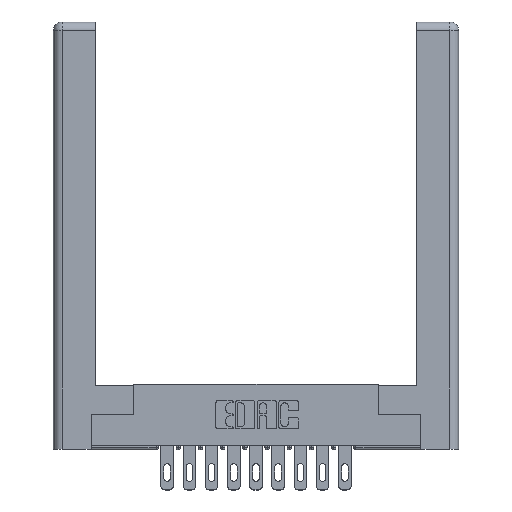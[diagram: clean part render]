
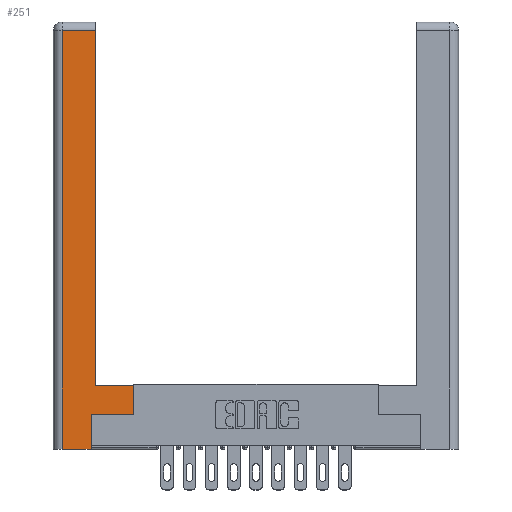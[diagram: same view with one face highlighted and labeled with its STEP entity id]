
A CAD part, top view. The second image highlights one B-rep face of the part: STEP entity #251.
In plain terms, the highlighted planar face has unit normal (0, 0, 1).
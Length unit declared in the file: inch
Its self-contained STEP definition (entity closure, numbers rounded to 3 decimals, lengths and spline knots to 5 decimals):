
#2 = CARTESIAN_POINT ( 'NONE',  ( 0.295, 2.94, 0. ) ) ;
#180 = LINE ( 'NONE', #5169, #15647 ) ;
#183 = VECTOR ( 'NONE', #11519, 39.37008 ) ;
#235 = CARTESIAN_POINT ( 'NONE',  ( 0.295, 0.45, 0. ) ) ;
#251 = ADVANCED_FACE ( 'NONE', ( #11973 ), #15130, .F. ) ;
#469 = ORIENTED_EDGE ( 'NONE', *, *, #1820, .T. ) ;
#1002 = CARTESIAN_POINT ( 'NONE',  ( 0.295, 3., 0. ) ) ;
#1596 = DIRECTION ( 'NONE',  ( -1., 0., 0. ) ) ;
#1722 = VECTOR ( 'NONE', #6594, 39.37008 ) ;
#1820 = EDGE_CURVE ( 'NONE', #2522, #3444, #8547, .T. ) ;
#1984 = ORIENTED_EDGE ( 'NONE', *, *, #8092, .T. ) ;
#2048 = LINE ( 'NONE', #10613, #3223 ) ;
#2414 = AXIS2_PLACEMENT_3D ( 'NONE', #3812, #12679, #1596 ) ;
#2522 = VERTEX_POINT ( 'NONE', #16158 ) ;
#2743 = CARTESIAN_POINT ( 'NONE',  ( 0.565, 0.245, 0. ) ) ;
#3223 = VECTOR ( 'NONE', #11830, 39.37008 ) ;
#3444 = VERTEX_POINT ( 'NONE', #5634 ) ;
#3812 = CARTESIAN_POINT ( 'NONE',  ( 0., 0., 0. ) ) ;
#4059 = CARTESIAN_POINT ( 'NONE',  ( 0.565, 0.245, 0. ) ) ;
#4212 = CARTESIAN_POINT ( 'NONE',  ( 0.265, 0., 0. ) ) ;
#4307 = VERTEX_POINT ( 'NONE', #4212 ) ;
#4383 = VERTEX_POINT ( 'NONE', #8502 ) ;
#4466 = VECTOR ( 'NONE', #4610, 39.37008 ) ;
#4610 = DIRECTION ( 'NONE',  ( 0., -1., 0. ) ) ;
#4736 = LINE ( 'NONE', #1002, #183 ) ;
#5169 = CARTESIAN_POINT ( 'NONE',  ( 0.265, 0.245, 0. ) ) ;
#5181 = VECTOR ( 'NONE', #12913, 39.37008 ) ;
#5294 = ORIENTED_EDGE ( 'NONE', *, *, #11824, .T. ) ;
#5634 = CARTESIAN_POINT ( 'NONE',  ( 0.295, 0.45, 0. ) ) ;
#6111 = CARTESIAN_POINT ( 'NONE',  ( 0.265, 0.245, 0. ) ) ;
#6594 = DIRECTION ( 'NONE',  ( 1., 0., 0. ) ) ;
#6601 = EDGE_CURVE ( 'NONE', #15083, #8939, #7186, .T. ) ;
#6635 = ORIENTED_EDGE ( 'NONE', *, *, #14468, .T. ) ;
#7186 = LINE ( 'NONE', #11523, #10351 ) ;
#7623 = DIRECTION ( 'NONE',  ( 0., 1., 0. ) ) ;
#7691 = DIRECTION ( 'NONE',  ( -1., 0., 0. ) ) ;
#7949 = ORIENTED_EDGE ( 'NONE', *, *, #11051, .T. ) ;
#7957 = ORIENTED_EDGE ( 'NONE', *, *, #10125, .T. ) ;
#8092 = EDGE_CURVE ( 'NONE', #3444, #15083, #4736, .T. ) ;
#8216 = VERTEX_POINT ( 'NONE', #6111 ) ;
#8502 = CARTESIAN_POINT ( 'NONE',  ( 0.0615, 0., 0. ) ) ;
#8547 = LINE ( 'NONE', #235, #5181 ) ;
#8631 = ORIENTED_EDGE ( 'NONE', *, *, #6601, .T. ) ;
#8854 = CARTESIAN_POINT ( 'NONE',  ( 0.565, 0.45, 0. ) ) ;
#8939 = VERTEX_POINT ( 'NONE', #10294 ) ;
#9630 = VERTEX_POINT ( 'NONE', #4059 ) ;
#10125 = EDGE_CURVE ( 'NONE', #8939, #4383, #14371, .T. ) ;
#10294 = CARTESIAN_POINT ( 'NONE',  ( 0.0615, 2.94, 0. ) ) ;
#10351 = VECTOR ( 'NONE', #7691, 39.37008 ) ;
#10606 = LINE ( 'NONE', #8854, #13576 ) ;
#10613 = CARTESIAN_POINT ( 'NONE',  ( 0.265, 0., 0. ) ) ;
#11051 = EDGE_CURVE ( 'NONE', #9630, #2522, #10606, .T. ) ;
#11327 = DIRECTION ( 'NONE',  ( 0., 1., 0. ) ) ;
#11519 = DIRECTION ( 'NONE',  ( 0., 1., 0. ) ) ;
#11523 = CARTESIAN_POINT ( 'NONE',  ( 0.0615, 2.94, 0. ) ) ;
#11824 = EDGE_CURVE ( 'NONE', #4383, #4307, #2048, .T. ) ;
#11830 = DIRECTION ( 'NONE',  ( 1., 0., 0. ) ) ;
#11973 = FACE_OUTER_BOUND ( 'NONE', #13375, .T. ) ;
#12679 = DIRECTION ( 'NONE',  ( 0., 0., -1. ) ) ;
#12913 = DIRECTION ( 'NONE',  ( -1., 0., 0. ) ) ;
#13375 = EDGE_LOOP ( 'NONE', ( #1984, #8631, #7957, #5294, #6635, #15597, #7949, #469 ) ) ;
#13576 = VECTOR ( 'NONE', #7623, 39.37008 ) ;
#14371 = LINE ( 'NONE', #15985, #4466 ) ;
#14468 = EDGE_CURVE ( 'NONE', #4307, #8216, #180, .T. ) ;
#15083 = VERTEX_POINT ( 'NONE', #2 ) ;
#15130 = PLANE ( 'NONE',  #2414 ) ;
#15215 = LINE ( 'NONE', #2743, #1722 ) ;
#15597 = ORIENTED_EDGE ( 'NONE', *, *, #16123, .T. ) ;
#15647 = VECTOR ( 'NONE', #11327, 39.37008 ) ;
#15985 = CARTESIAN_POINT ( 'NONE',  ( 0.0615, 0., 0. ) ) ;
#16123 = EDGE_CURVE ( 'NONE', #8216, #9630, #15215, .T. ) ;
#16158 = CARTESIAN_POINT ( 'NONE',  ( 0.565, 0.45, 0. ) ) ;
